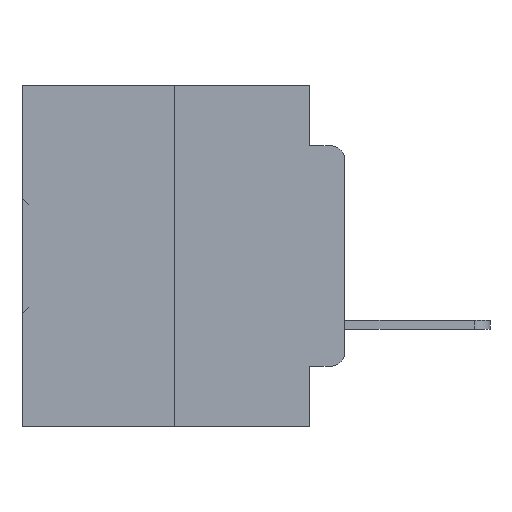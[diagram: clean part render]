
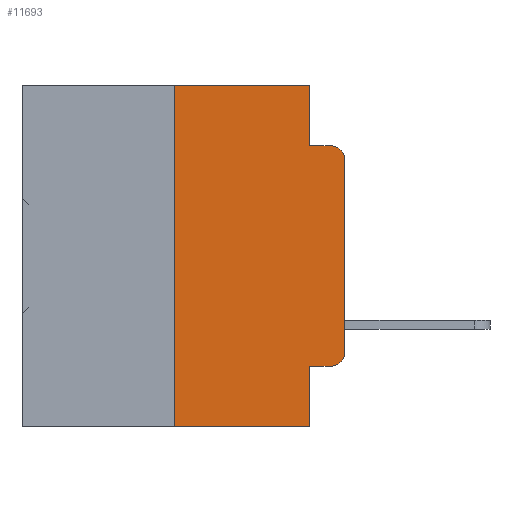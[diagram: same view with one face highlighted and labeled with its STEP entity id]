
A CAD part, left-side view. The second image highlights one B-rep face of the part: STEP entity #11693.
In plain terms, the highlighted planar face has unit normal (-1, 0, 0).
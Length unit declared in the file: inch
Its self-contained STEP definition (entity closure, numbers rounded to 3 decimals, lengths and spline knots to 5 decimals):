
#484 = VERTEX_POINT ( 'NONE', #35715 ) ;
#587 = AXIS2_PLACEMENT_3D ( 'NONE', #16212, #35512, #19094 ) ;
#739 = CARTESIAN_POINT ( 'NONE',  ( 0., 0.051, -0.5 ) ) ;
#1096 = EDGE_CURVE ( 'NONE', #28204, #11936, #21033, .T. ) ;
#1234 = VECTOR ( 'NONE', #28343, 39.37008 ) ;
#1548 = DIRECTION ( 'NONE',  ( 1., 0., 0. ) ) ;
#2013 = ORIENTED_EDGE ( 'NONE', *, *, #15510, .T. ) ;
#2746 = CARTESIAN_POINT ( 'NONE',  ( 0., 0.02, -0.4115 ) ) ;
#3213 = CARTESIAN_POINT ( 'NONE',  ( 0., 0.25, 0. ) ) ;
#3304 = CARTESIAN_POINT ( 'NONE',  ( 0., 0.02, -0.0885 ) ) ;
#3369 = VECTOR ( 'NONE', #34508, 39.37008 ) ;
#3514 = EDGE_LOOP ( 'NONE', ( #13265, #20904, #22642, #28680, #35859, #23092, #8592, #29942, #9083, #2013 ) ) ;
#4261 = EDGE_CURVE ( 'NONE', #17120, #15262, #24751, .T. ) ;
#4334 = LINE ( 'NONE', #3213, #3369 ) ;
#5126 = VECTOR ( 'NONE', #9287, 39.37008 ) ;
#5359 = CARTESIAN_POINT ( 'NONE',  ( 0., 0.473, 0. ) ) ;
#6298 = CARTESIAN_POINT ( 'NONE',  ( 0., 0.051, 0. ) ) ;
#6326 = EDGE_CURVE ( 'NONE', #8292, #13658, #9283, .T. ) ;
#6758 = EDGE_CURVE ( 'NONE', #11936, #17930, #31874, .T. ) ;
#7379 = LINE ( 'NONE', #31319, #36435 ) ;
#7542 = LINE ( 'NONE', #13475, #21246 ) ;
#7767 = EDGE_CURVE ( 'NONE', #484, #17930, #7379, .T. ) ;
#8116 = CIRCLE ( 'NONE', #28067, 0.02 ) ;
#8292 = VERTEX_POINT ( 'NONE', #8342 ) ;
#8342 = CARTESIAN_POINT ( 'NONE',  ( 0., 0.25, 0. ) ) ;
#8592 = ORIENTED_EDGE ( 'NONE', *, *, #33544, .T. ) ;
#9083 = ORIENTED_EDGE ( 'NONE', *, *, #12352, .T. ) ;
#9283 = LINE ( 'NONE', #5359, #1234 ) ;
#9287 = DIRECTION ( 'NONE',  ( 0., 0., -1. ) ) ;
#9496 = CARTESIAN_POINT ( 'NONE',  ( 0., 0.051, -0.4115 ) ) ;
#10024 = DIRECTION ( 'NONE',  ( 0., 0., 1. ) ) ;
#11693 = ADVANCED_FACE ( 'NONE', ( #24313 ), #19297, .F. ) ;
#11936 = VERTEX_POINT ( 'NONE', #31327 ) ;
#12352 = EDGE_CURVE ( 'NONE', #17120, #27968, #7542, .T. ) ;
#12871 = CARTESIAN_POINT ( 'NONE',  ( 0., 0., -0.3915 ) ) ;
#13265 = ORIENTED_EDGE ( 'NONE', *, *, #1096, .T. ) ;
#13475 = CARTESIAN_POINT ( 'NONE',  ( 0., 0.051, -0.4115 ) ) ;
#13658 = VERTEX_POINT ( 'NONE', #14182 ) ;
#14066 = CARTESIAN_POINT ( 'NONE',  ( 0., 0.473, -0.5 ) ) ;
#14182 = CARTESIAN_POINT ( 'NONE',  ( 0., 0.051, 0. ) ) ;
#14662 = DIRECTION ( 'NONE',  ( 0., -1., 0. ) ) ;
#14803 = VECTOR ( 'NONE', #19586, 39.37008 ) ;
#14943 = DIRECTION ( 'NONE',  ( 0., 0., -1. ) ) ;
#15241 = CARTESIAN_POINT ( 'NONE',  ( 0., 0., 0. ) ) ;
#15262 = VERTEX_POINT ( 'NONE', #739 ) ;
#15510 = EDGE_CURVE ( 'NONE', #27968, #28204, #8116, .T. ) ;
#16212 = CARTESIAN_POINT ( 'NONE',  ( 0., 0.02, -0.1085 ) ) ;
#16956 = DIRECTION ( 'NONE',  ( -1., 0., 0. ) ) ;
#17120 = VERTEX_POINT ( 'NONE', #9496 ) ;
#17930 = VERTEX_POINT ( 'NONE', #3304 ) ;
#19094 = DIRECTION ( 'NONE',  ( 0., 0., -1. ) ) ;
#19297 = PLANE ( 'NONE',  #24293 ) ;
#19586 = DIRECTION ( 'NONE',  ( 0., -1., 0. ) ) ;
#20904 = ORIENTED_EDGE ( 'NONE', *, *, #6758, .T. ) ;
#21033 = LINE ( 'NONE', #15241, #36384 ) ;
#21246 = VECTOR ( 'NONE', #21973, 39.37008 ) ;
#21973 = DIRECTION ( 'NONE',  ( 0., -1., 0. ) ) ;
#22138 = DIRECTION ( 'NONE',  ( 0., 0., -1. ) ) ;
#22642 = ORIENTED_EDGE ( 'NONE', *, *, #7767, .F. ) ;
#23092 = ORIENTED_EDGE ( 'NONE', *, *, #36080, .F. ) ;
#24293 = AXIS2_PLACEMENT_3D ( 'NONE', #30264, #1548, #22138 ) ;
#24313 = FACE_OUTER_BOUND ( 'NONE', #3514, .T. ) ;
#24751 = LINE ( 'NONE', #31598, #36636 ) ;
#27968 = VERTEX_POINT ( 'NONE', #2746 ) ;
#28067 = AXIS2_PLACEMENT_3D ( 'NONE', #33479, #16956, #36186 ) ;
#28079 = LINE ( 'NONE', #6298, #5126 ) ;
#28204 = VERTEX_POINT ( 'NONE', #12871 ) ;
#28343 = DIRECTION ( 'NONE',  ( 0., -1., 0. ) ) ;
#28680 = ORIENTED_EDGE ( 'NONE', *, *, #32468, .F. ) ;
#29942 = ORIENTED_EDGE ( 'NONE', *, *, #4261, .F. ) ;
#30264 = CARTESIAN_POINT ( 'NONE',  ( 0., 0.473, 0. ) ) ;
#31319 = CARTESIAN_POINT ( 'NONE',  ( 0., 0.051, -0.0885 ) ) ;
#31327 = CARTESIAN_POINT ( 'NONE',  ( 0., 0., -0.1085 ) ) ;
#31598 = CARTESIAN_POINT ( 'NONE',  ( 0., 0.051, 0. ) ) ;
#31874 = CIRCLE ( 'NONE', #587, 0.02 ) ;
#32236 = VERTEX_POINT ( 'NONE', #36158 ) ;
#32468 = EDGE_CURVE ( 'NONE', #13658, #484, #28079, .T. ) ;
#33479 = CARTESIAN_POINT ( 'NONE',  ( 0., 0.02, -0.3915 ) ) ;
#33544 = EDGE_CURVE ( 'NONE', #32236, #15262, #35970, .T. ) ;
#34508 = DIRECTION ( 'NONE',  ( 0., 0., 1. ) ) ;
#35512 = DIRECTION ( 'NONE',  ( -1., 0., 0. ) ) ;
#35715 = CARTESIAN_POINT ( 'NONE',  ( 0., 0.051, -0.0885 ) ) ;
#35859 = ORIENTED_EDGE ( 'NONE', *, *, #6326, .F. ) ;
#35970 = LINE ( 'NONE', #14066, #14803 ) ;
#36080 = EDGE_CURVE ( 'NONE', #32236, #8292, #4334, .T. ) ;
#36158 = CARTESIAN_POINT ( 'NONE',  ( 0., 0.25, -0.5 ) ) ;
#36186 = DIRECTION ( 'NONE',  ( 0., 0., -1. ) ) ;
#36384 = VECTOR ( 'NONE', #10024, 39.37008 ) ;
#36435 = VECTOR ( 'NONE', #14662, 39.37008 ) ;
#36636 = VECTOR ( 'NONE', #14943, 39.37008 ) ;
